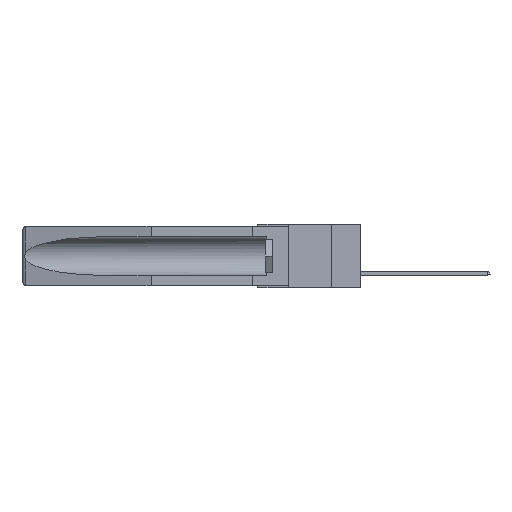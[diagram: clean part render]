
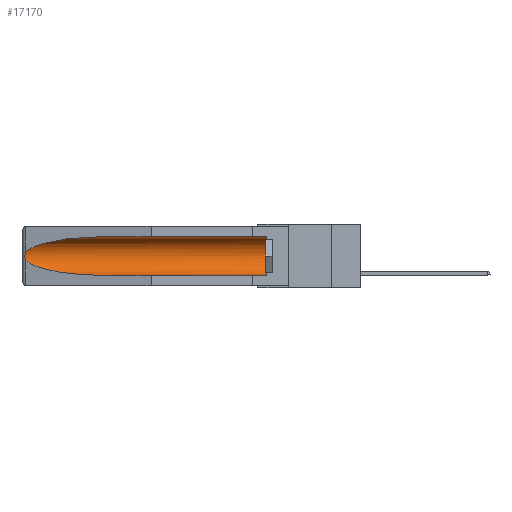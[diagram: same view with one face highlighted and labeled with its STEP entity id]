
A CAD part, left-side view. The second image highlights one B-rep face of the part: STEP entity #17170.
In plain terms, the highlighted cylindrical face has radius 2.857 mm (diameter 5.715 mm), a partial arc.
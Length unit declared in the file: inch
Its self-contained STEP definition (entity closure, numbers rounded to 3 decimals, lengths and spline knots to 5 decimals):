
#64 = VECTOR ( 'NONE', #13586, 39.37008 ) ;
#291 = CARTESIAN_POINT ( 'NONE',  ( 0.26597, 1.52961, -0.15275 ) ) ;
#602 = ORIENTED_EDGE ( 'NONE', *, *, #1410, .T. ) ;
#864 = AXIS2_PLACEMENT_3D ( 'NONE', #11441, #3144, #11516 ) ;
#1410 = EDGE_CURVE ( 'NONE', #8346, #19171, #20802, .T. ) ;
#1824 =( BOUNDED_CURVE ( )  B_SPLINE_CURVE ( 3, ( #7600, #2516, #14057, #15809 ),
 .UNSPECIFIED., .F., .F. ) 
 B_SPLINE_CURVE_WITH_KNOTS ( ( 4, 4 ),
 ( 4.71239, 6.08839 ),
 .UNSPECIFIED. ) 
 CURVE ( )  GEOMETRIC_REPRESENTATION_ITEM ( )  RATIONAL_B_SPLINE_CURVE ( ( 1., 0.848, 0.848, 1. ) ) 
 REPRESENTATION_ITEM ( '' )  );
#1971 = CARTESIAN_POINT ( 'NONE',  ( 0.155, -0.30754, -0.059 ) ) ;
#2043 = ORIENTED_EDGE ( 'NONE', *, *, #7414, .F. ) ;
#2516 = CARTESIAN_POINT ( 'NONE',  ( 0.21114, 1.30732, -0.059 ) ) ;
#2841 = CARTESIAN_POINT ( 'NONE',  ( 0.25451, 1.48313, -0.24835 ) ) ;
#2888 = VERTEX_POINT ( 'NONE', #14296 ) ;
#3036 = CARTESIAN_POINT ( 'NONE',  ( 0.155, 0.126, -0.284 ) ) ;
#3144 = DIRECTION ( 'NONE',  ( 0., 1., 0. ) ) ;
#3284 = VERTEX_POINT ( 'NONE', #6561 ) ;
#3733 = CARTESIAN_POINT ( 'NONE',  ( 0.2675, 1.53308, -0.17534 ) ) ;
#3805 = CARTESIAN_POINT ( 'NONE',  ( 0.2673, 1.5327, -0.16383 ) ) ;
#4856 = CARTESIAN_POINT ( 'NONE',  ( 0.155, 0.126, -0.1715 ) ) ;
#5116 = ORIENTED_EDGE ( 'NONE', *, *, #12247, .T. ) ;
#6227 = CARTESIAN_POINT ( 'NONE',  ( 0.155, -0.30754, -0.284 ) ) ;
#6561 = CARTESIAN_POINT ( 'NONE',  ( 0.26537, 1.52718, -0.14972 ) ) ;
#6647 = CARTESIAN_POINT ( 'NONE',  ( 0.155, 1.07973, -0.059 ) ) ;
#7414 = EDGE_CURVE ( 'NONE', #12665, #19171, #8825, .T. ) ;
#7578 = EDGE_LOOP ( 'NONE', ( #14710, #5116, #602, #2043, #9660, #20908 ) ) ;
#7600 = CARTESIAN_POINT ( 'NONE',  ( 0.155, 1.07973, -0.059 ) ) ;
#8115 = DIRECTION ( 'NONE',  ( 0., -1., 0. ) ) ;
#8346 = VERTEX_POINT ( 'NONE', #20280 ) ;
#8799 = EDGE_CURVE ( 'NONE', #12665, #2888, #16868, .T. ) ;
#8825 = LINE ( 'NONE', #6227, #18715 ) ;
#9474 = VERTEX_POINT ( 'NONE', #6647 ) ;
#9549 = AXIS2_PLACEMENT_3D ( 'NONE', #4856, #8115, #11631 ) ;
#9660 = ORIENTED_EDGE ( 'NONE', *, *, #8799, .T. ) ;
#9904 = EDGE_CURVE ( 'NONE', #9474, #3284, #1824, .T. ) ;
#10352 = CARTESIAN_POINT ( 'NONE',  ( 0.26654, 1.53092, -0.15636 ) ) ;
#11441 = CARTESIAN_POINT ( 'NONE',  ( 0.155, -0.30754, -0.1715 ) ) ;
#11516 = DIRECTION ( 'NONE',  ( 0., 0., 1. ) ) ;
#11631 = DIRECTION ( 'NONE',  ( 0., 0., 1. ) ) ;
#12023 = CARTESIAN_POINT ( 'NONE',  ( 0.26537, 1.52718, -0.19328 ) ) ;
#12247 = EDGE_CURVE ( 'NONE', #3284, #8346, #17308, .T. ) ;
#12665 = VERTEX_POINT ( 'NONE', #3036 ) ;
#12704 = CARTESIAN_POINT ( 'NONE',  ( 0.26537, 1.52718, -0.19328 ) ) ;
#12777 = CARTESIAN_POINT ( 'NONE',  ( 0.21114, 1.30732, -0.284 ) ) ;
#13530 = CARTESIAN_POINT ( 'NONE',  ( 0.2675, 1.53308, -0.16763 ) ) ;
#13586 = DIRECTION ( 'NONE',  ( 0., 1., 0. ) ) ;
#13682 = EDGE_CURVE ( 'NONE', #2888, #9474, #20635, .T. ) ;
#14057 = CARTESIAN_POINT ( 'NONE',  ( 0.25451, 1.48313, -0.09465 ) ) ;
#14296 = CARTESIAN_POINT ( 'NONE',  ( 0.155, 0.126, -0.059 ) ) ;
#14659 = DIRECTION ( 'NONE',  ( 0., 1., 0. ) ) ;
#14710 = ORIENTED_EDGE ( 'NONE', *, *, #9904, .T. ) ;
#15281 = CARTESIAN_POINT ( 'NONE',  ( 0.26597, 1.5296, -0.19026 ) ) ;
#15424 = CARTESIAN_POINT ( 'NONE',  ( 0.2673, 1.53269, -0.17917 ) ) ;
#15809 = CARTESIAN_POINT ( 'NONE',  ( 0.26537, 1.52718, -0.14972 ) ) ;
#15985 = CARTESIAN_POINT ( 'NONE',  ( 0.155, 1.07973, -0.284 ) ) ;
#16868 = CIRCLE ( 'NONE', #9549, 0.1125 ) ;
#17170 = ADVANCED_FACE ( 'NONE', ( #18662 ), #19984, .F. ) ;
#17308 = B_SPLINE_CURVE_WITH_KNOTS ( 'NONE', 3,
 ( #18546, #291, #10352, #3805, #13530, #3733, #15424, #20371, #15281, #12023 ),
 .UNSPECIFIED., .F., .F.,
 ( 4, 2, 2, 2, 4 ),
 ( 0., 0.00029, 0.00058, 0.00087, 0.00117 ),
 .UNSPECIFIED. ) ;
#18546 = CARTESIAN_POINT ( 'NONE',  ( 0.26537, 1.52718, -0.14972 ) ) ;
#18662 = FACE_OUTER_BOUND ( 'NONE', #7578, .T. ) ;
#18715 = VECTOR ( 'NONE', #14659, 39.37008 ) ;
#19171 = VERTEX_POINT ( 'NONE', #20432 ) ;
#19984 = CYLINDRICAL_SURFACE ( 'NONE', #864, 0.1125 ) ;
#20280 = CARTESIAN_POINT ( 'NONE',  ( 0.26537, 1.52718, -0.19328 ) ) ;
#20371 = CARTESIAN_POINT ( 'NONE',  ( 0.26655, 1.53094, -0.18657 ) ) ;
#20432 = CARTESIAN_POINT ( 'NONE',  ( 0.155, 1.07973, -0.284 ) ) ;
#20635 = LINE ( 'NONE', #1971, #64 ) ;
#20802 =( BOUNDED_CURVE ( )  B_SPLINE_CURVE ( 3, ( #12704, #2841, #12777, #15985 ),
 .UNSPECIFIED., .F., .F. ) 
 B_SPLINE_CURVE_WITH_KNOTS ( ( 4, 4 ),
 ( 0.1948, 1.5708 ),
 .UNSPECIFIED. ) 
 CURVE ( )  GEOMETRIC_REPRESENTATION_ITEM ( )  RATIONAL_B_SPLINE_CURVE ( ( 1., 0.848, 0.848, 1. ) ) 
 REPRESENTATION_ITEM ( '' )  );
#20908 = ORIENTED_EDGE ( 'NONE', *, *, #13682, .T. ) ;
